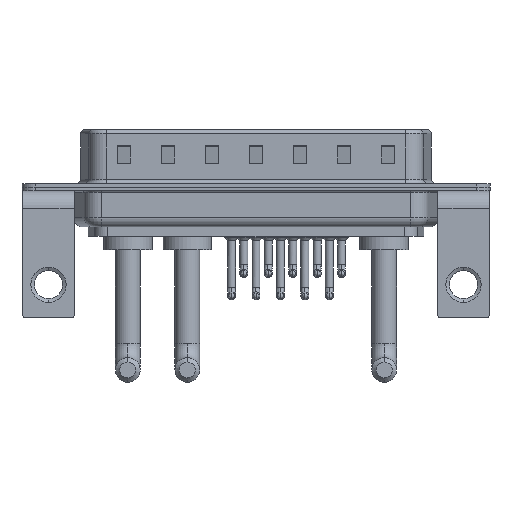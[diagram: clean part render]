
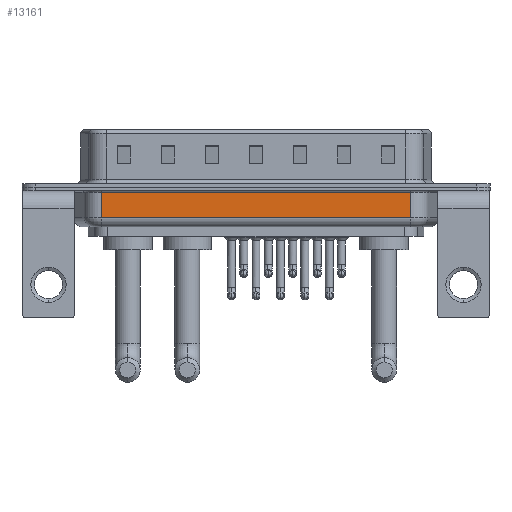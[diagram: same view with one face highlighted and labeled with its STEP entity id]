
A CAD part, front view. The second image highlights one B-rep face of the part: STEP entity #13161.
In plain terms, the highlighted planar face has unit normal (0, -1, 0).
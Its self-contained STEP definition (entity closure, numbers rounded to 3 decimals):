
#869 = AXIS2_PLACEMENT_3D ( 'NONE', #7793, #19662, #17572 ) ;
#1077 = VERTEX_POINT ( 'NONE', #21017 ) ;
#2424 = LINE ( 'NONE', #10013, #7224 ) ;
#2650 = DIRECTION ( 'NONE',  ( 0., 0., 1. ) ) ;
#3126 = VECTOR ( 'NONE', #19840, 1000. ) ;
#3652 = CARTESIAN_POINT ( 'NONE',  ( 6.006, -5.35, -0.65 ) ) ;
#5227 = ORIENTED_EDGE ( 'NONE', *, *, #9962, .T. ) ;
#5525 = VERTEX_POINT ( 'NONE', #3652 ) ;
#6615 = LINE ( 'NONE', #12279, #3126 ) ;
#6934 = DIRECTION ( 'NONE',  ( -1., 0., 0. ) ) ;
#7165 = LINE ( 'NONE', #18317, #15371 ) ;
#7224 = VECTOR ( 'NONE', #17578, 1000. ) ;
#7350 = EDGE_LOOP ( 'NONE', ( #18853, #5227, #20451, #15901 ) ) ;
#7793 = CARTESIAN_POINT ( 'NONE',  ( 6.006, -5.35, -4.5 ) ) ;
#9078 = EDGE_CURVE ( 'NONE', #1077, #5525, #7165, .T. ) ;
#9946 = CARTESIAN_POINT ( 'NONE',  ( 41.044, -5.35, -3.5 ) ) ;
#9962 = EDGE_CURVE ( 'NONE', #16229, #20576, #6615, .T. ) ;
#10013 = CARTESIAN_POINT ( 'NONE',  ( 6.006, -5.35, -4.5 ) ) ;
#12279 = CARTESIAN_POINT ( 'NONE',  ( 6.006, -5.35, -3.5 ) ) ;
#13161 = ADVANCED_FACE ( 'NONE', ( #19416 ), #23138, .F. ) ;
#14532 = EDGE_CURVE ( 'NONE', #16229, #5525, #2424, .T. ) ;
#15371 = VECTOR ( 'NONE', #6934, 1000. ) ;
#15901 = ORIENTED_EDGE ( 'NONE', *, *, #9078, .T. ) ;
#16229 = VERTEX_POINT ( 'NONE', #17556 ) ;
#17556 = CARTESIAN_POINT ( 'NONE',  ( 6.006, -5.35, -3.5 ) ) ;
#17572 = DIRECTION ( 'NONE',  ( 0., 0., 1. ) ) ;
#17578 = DIRECTION ( 'NONE',  ( 0., 0., 1. ) ) ;
#17786 = LINE ( 'NONE', #21246, #23562 ) ;
#18317 = CARTESIAN_POINT ( 'NONE',  ( 6.006, -5.35, -0.65 ) ) ;
#18853 = ORIENTED_EDGE ( 'NONE', *, *, #14532, .F. ) ;
#19416 = FACE_OUTER_BOUND ( 'NONE', #7350, .T. ) ;
#19662 = DIRECTION ( 'NONE',  ( 0., 1., 0. ) ) ;
#19840 = DIRECTION ( 'NONE',  ( 1., 0., 0. ) ) ;
#20451 = ORIENTED_EDGE ( 'NONE', *, *, #24308, .T. ) ;
#20576 = VERTEX_POINT ( 'NONE', #9946 ) ;
#21017 = CARTESIAN_POINT ( 'NONE',  ( 41.044, -5.35, -0.65 ) ) ;
#21246 = CARTESIAN_POINT ( 'NONE',  ( 41.044, -5.35, -4.5 ) ) ;
#23138 = PLANE ( 'NONE',  #869 ) ;
#23562 = VECTOR ( 'NONE', #2650, 1000. ) ;
#24308 = EDGE_CURVE ( 'NONE', #20576, #1077, #17786, .T. ) ;
